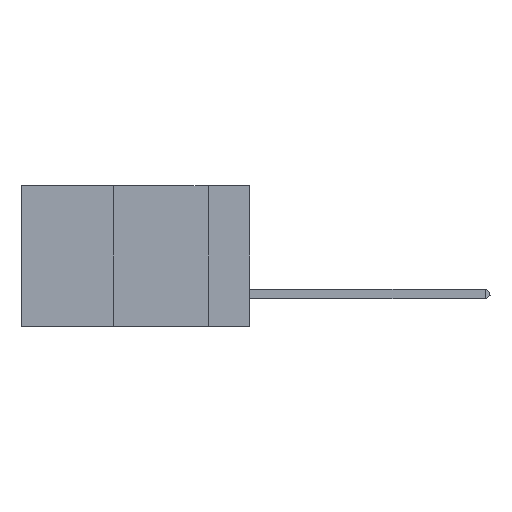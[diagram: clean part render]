
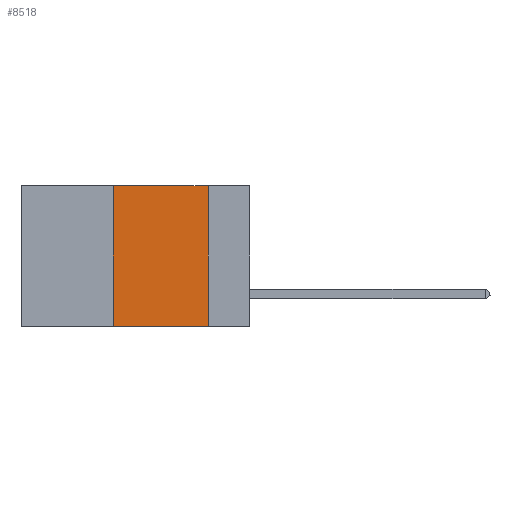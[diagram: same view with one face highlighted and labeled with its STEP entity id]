
A CAD part, left-side view. The second image highlights one B-rep face of the part: STEP entity #8518.
In plain terms, the highlighted planar face has unit normal (-1, 0, 0).
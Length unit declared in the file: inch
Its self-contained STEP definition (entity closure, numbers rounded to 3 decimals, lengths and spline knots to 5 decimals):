
#655 = ORIENTED_EDGE ( 'NONE', *, *, #24847, .F. ) ;
#3611 = VECTOR ( 'NONE', #21207, 39.37008 ) ;
#3618 = PLANE ( 'NONE',  #19511 ) ;
#4419 = LINE ( 'NONE', #36095, #16102 ) ;
#4602 = LINE ( 'NONE', #17897, #13636 ) ;
#6203 = CARTESIAN_POINT ( 'NONE',  ( 0., 0.36, 0. ) ) ;
#6839 = LINE ( 'NONE', #13872, #25714 ) ;
#7573 = CARTESIAN_POINT ( 'NONE',  ( 0., 0.11, 0. ) ) ;
#8518 = ADVANCED_FACE ( 'NONE', ( #29732 ), #3618, .F. ) ;
#9829 = ORIENTED_EDGE ( 'NONE', *, *, #20577, .F. ) ;
#12372 = CARTESIAN_POINT ( 'NONE',  ( 0., 0.36, 0. ) ) ;
#12905 = VERTEX_POINT ( 'NONE', #26105 ) ;
#13237 = ORIENTED_EDGE ( 'NONE', *, *, #36110, .T. ) ;
#13636 = VECTOR ( 'NONE', #32546, 39.37008 ) ;
#13872 = CARTESIAN_POINT ( 'NONE',  ( 0., 0.6, -0.37 ) ) ;
#14699 = ORIENTED_EDGE ( 'NONE', *, *, #32579, .F. ) ;
#16102 = VECTOR ( 'NONE', #33211, 39.37008 ) ;
#17897 = CARTESIAN_POINT ( 'NONE',  ( 0., 0.11, 0. ) ) ;
#19511 = AXIS2_PLACEMENT_3D ( 'NONE', #23491, #32079, #29583 ) ;
#20577 = EDGE_CURVE ( 'NONE', #31624, #28022, #23862, .T. ) ;
#21207 = DIRECTION ( 'NONE',  ( 0., 0., 1. ) ) ;
#23491 = CARTESIAN_POINT ( 'NONE',  ( 0., 0.6, 0. ) ) ;
#23862 = LINE ( 'NONE', #12372, #3611 ) ;
#24579 = EDGE_LOOP ( 'NONE', ( #655, #14699, #9829, #13237 ) ) ;
#24847 = EDGE_CURVE ( 'NONE', #29539, #12905, #4602, .T. ) ;
#25320 = DIRECTION ( 'NONE',  ( 0., -1., 0. ) ) ;
#25714 = VECTOR ( 'NONE', #25320, 39.37008 ) ;
#26105 = CARTESIAN_POINT ( 'NONE',  ( 0., 0.11, -0.37 ) ) ;
#26612 = CARTESIAN_POINT ( 'NONE',  ( 0., 0.36, -0.37 ) ) ;
#28022 = VERTEX_POINT ( 'NONE', #6203 ) ;
#29539 = VERTEX_POINT ( 'NONE', #7573 ) ;
#29583 = DIRECTION ( 'NONE',  ( 0., 0., -1. ) ) ;
#29732 = FACE_OUTER_BOUND ( 'NONE', #24579, .T. ) ;
#31624 = VERTEX_POINT ( 'NONE', #26612 ) ;
#32079 = DIRECTION ( 'NONE',  ( 1., 0., 0. ) ) ;
#32546 = DIRECTION ( 'NONE',  ( 0., 0., -1. ) ) ;
#32579 = EDGE_CURVE ( 'NONE', #28022, #29539, #4419, .T. ) ;
#33211 = DIRECTION ( 'NONE',  ( 0., -1., 0. ) ) ;
#36095 = CARTESIAN_POINT ( 'NONE',  ( 0., 0.6, 0. ) ) ;
#36110 = EDGE_CURVE ( 'NONE', #31624, #12905, #6839, .T. ) ;
